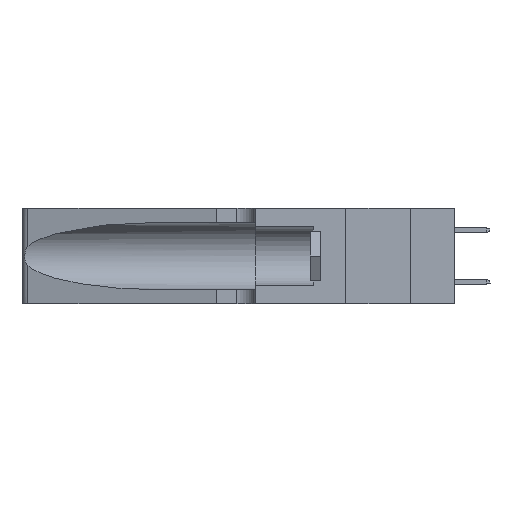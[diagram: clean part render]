
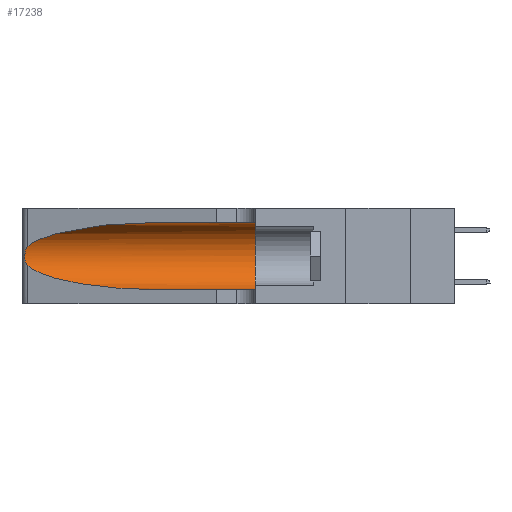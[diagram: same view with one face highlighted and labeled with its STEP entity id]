
A CAD part, left-side view. The second image highlights one B-rep face of the part: STEP entity #17238.
In plain terms, the highlighted cylindrical face has radius 3.308 mm (diameter 6.617 mm), a partial arc.
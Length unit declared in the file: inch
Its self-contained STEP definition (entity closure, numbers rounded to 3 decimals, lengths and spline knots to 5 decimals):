
#310 = CARTESIAN_POINT ( 'NONE',  ( 0.1305, 1.61858, 0.185 ) ) ;
#352 = CARTESIAN_POINT ( 'NONE',  ( 0.25487, 1.22718, 0.22369 ) ) ;
#636 = DIRECTION ( 'NONE',  ( 0., 1., 0. ) ) ;
#2686 = DIRECTION ( 'NONE',  ( 0., 0., 1. ) ) ;
#3085 = EDGE_CURVE ( 'NONE', #28419, #7694, #16352, .T. ) ;
#3163 = EDGE_LOOP ( 'NONE', ( #8327, #13606, #5145, #22770, #24645, #8118 ) ) ;
#3360 = CARTESIAN_POINT ( 'NONE',  ( 0.26075, 1.23896, 0.178 ) ) ;
#3658 = CARTESIAN_POINT ( 'NONE',  ( 0.25487, 1.22718, 0.22369 ) ) ;
#3669 = AXIS2_PLACEMENT_3D ( 'NONE', #310, #9234, #22348 ) ;
#4435 = CARTESIAN_POINT ( 'NONE',  ( 0.25487, 1.22718, 0.14631 ) ) ;
#5102 = EDGE_CURVE ( 'NONE', #12099, #28419, #13358, .T. ) ;
#5145 = ORIENTED_EDGE ( 'NONE', *, *, #10471, .T. ) ;
#7182 = CARTESIAN_POINT ( 'NONE',  ( 0.25555, 1.22994, 0.2215 ) ) ;
#7206 = CARTESIAN_POINT ( 'NONE',  ( 0.1305, 0.35, 0.185 ) ) ;
#7694 = VERTEX_POINT ( 'NONE', #22421 ) ;
#7907 = CARTESIAN_POINT ( 'NONE',  ( 0.1305, 0.72297, 0.31525 ) ) ;
#8118 = ORIENTED_EDGE ( 'NONE', *, *, #5102, .F. ) ;
#8327 = ORIENTED_EDGE ( 'NONE', *, *, #25063, .T. ) ;
#8345 = VECTOR ( 'NONE', #12967, 39.37008 ) ;
#9234 = DIRECTION ( 'NONE',  ( 0., -1., 0. ) ) ;
#9275 = EDGE_CURVE ( 'NONE', #16780, #10342, #11968, .T. ) ;
#9394 = CARTESIAN_POINT ( 'NONE',  ( 0.25487, 1.22718, 0.14631 ) ) ;
#9401 = CARTESIAN_POINT ( 'NONE',  ( 0.25487, 1.22718, 0.22369 ) ) ;
#10110 = CARTESIAN_POINT ( 'NONE',  ( 0.26075, 1.23896, 0.19203 ) ) ;
#10342 = VERTEX_POINT ( 'NONE', #28223 ) ;
#10471 = EDGE_CURVE ( 'NONE', #10342, #26490, #19656, .T. ) ;
#11968 = B_SPLINE_CURVE_WITH_KNOTS ( 'NONE', 3,
 ( #9401, #7182, #14020, #18959, #14452, #23371, #10110, #3360, #27914, #12275, #18146, #15939, #22121, #4435 ),
 .UNSPECIFIED., .F., .F.,
 ( 4, 2, 2, 2, 2, 2, 4 ),
 ( 0., 0.00027, 0.00053, 0.00107, 0.0016, 0.00187, 0.00214 ),
 .UNSPECIFIED. ) ;
#12099 = VERTEX_POINT ( 'NONE', #7907 ) ;
#12275 = CARTESIAN_POINT ( 'NONE',  ( 0.25856, 1.23593, 0.16098 ) ) ;
#12567 = CARTESIAN_POINT ( 'NONE',  ( 0.1305, 0.72297, 0.31525 ) ) ;
#12763 =( BOUNDED_CURVE ( )  B_SPLINE_CURVE ( 3, ( #12567, #28210, #28356, #3658 ),
 .UNSPECIFIED., .F., .T. ) 
 B_SPLINE_CURVE_WITH_KNOTS ( ( 4, 4 ),
 ( 1.5708, 2.84003 ),
 .UNSPECIFIED. ) 
 CURVE ( )  GEOMETRIC_REPRESENTATION_ITEM ( )  RATIONAL_B_SPLINE_CURVE ( ( 1., 0.87, 0.87, 1. ) ) 
 REPRESENTATION_ITEM ( '' )  );
#12967 = DIRECTION ( 'NONE',  ( 0., -1., 0. ) ) ;
#13121 = LINE ( 'NONE', #28623, #8345 ) ;
#13358 = LINE ( 'NONE', #15959, #15844 ) ;
#13432 = CYLINDRICAL_SURFACE ( 'NONE', #3669, 0.13025 ) ;
#13606 = ORIENTED_EDGE ( 'NONE', *, *, #9275, .T. ) ;
#14020 = CARTESIAN_POINT ( 'NONE',  ( 0.25639, 1.23184, 0.21858 ) ) ;
#14452 = CARTESIAN_POINT ( 'NONE',  ( 0.25854, 1.2359, 0.20912 ) ) ;
#15586 = CARTESIAN_POINT ( 'NONE',  ( 0.1305, 0.35, 0.31525 ) ) ;
#15844 = VECTOR ( 'NONE', #27120, 39.37008 ) ;
#15939 = CARTESIAN_POINT ( 'NONE',  ( 0.25639, 1.23186, 0.15144 ) ) ;
#15959 = CARTESIAN_POINT ( 'NONE',  ( 0.1305, 1.61858, 0.31525 ) ) ;
#16352 = CIRCLE ( 'NONE', #27566, 0.13025 ) ;
#16780 = VERTEX_POINT ( 'NONE', #352 ) ;
#17238 = ADVANCED_FACE ( 'NONE', ( #24991 ), #13432, .F. ) ;
#18107 = CARTESIAN_POINT ( 'NONE',  ( 0.2373, 1.15595, 0.08982 ) ) ;
#18146 = CARTESIAN_POINT ( 'NONE',  ( 0.25789, 1.23486, 0.15765 ) ) ;
#18251 = CARTESIAN_POINT ( 'NONE',  ( 0.18966, 0.96281, 0.05475 ) ) ;
#18872 = EDGE_CURVE ( 'NONE', #26490, #7694, #13121, .T. ) ;
#18959 = CARTESIAN_POINT ( 'NONE',  ( 0.25787, 1.23484, 0.2124 ) ) ;
#19656 =( BOUNDED_CURVE ( )  B_SPLINE_CURVE ( 3, ( #9394, #18107, #18251, #27198 ),
 .UNSPECIFIED., .F., .T. ) 
 B_SPLINE_CURVE_WITH_KNOTS ( ( 4, 4 ),
 ( 3.44316, 4.71239 ),
 .UNSPECIFIED. ) 
 CURVE ( )  GEOMETRIC_REPRESENTATION_ITEM ( )  RATIONAL_B_SPLINE_CURVE ( ( 1., 0.87, 0.87, 1. ) ) 
 REPRESENTATION_ITEM ( '' )  );
#22121 = CARTESIAN_POINT ( 'NONE',  ( 0.25555, 1.22993, 0.14849 ) ) ;
#22348 = DIRECTION ( 'NONE',  ( 0., 0., -1. ) ) ;
#22421 = CARTESIAN_POINT ( 'NONE',  ( 0.1305, 0.35, 0.05475 ) ) ;
#22770 = ORIENTED_EDGE ( 'NONE', *, *, #18872, .T. ) ;
#23371 = CARTESIAN_POINT ( 'NONE',  ( 0.26018, 1.23835, 0.19895 ) ) ;
#24645 = ORIENTED_EDGE ( 'NONE', *, *, #3085, .F. ) ;
#24991 = FACE_OUTER_BOUND ( 'NONE', #3163, .T. ) ;
#25063 = EDGE_CURVE ( 'NONE', #12099, #16780, #12763, .T. ) ;
#25876 = CARTESIAN_POINT ( 'NONE',  ( 0.1305, 0.72297, 0.05475 ) ) ;
#26490 = VERTEX_POINT ( 'NONE', #25876 ) ;
#27120 = DIRECTION ( 'NONE',  ( 0., -1., 0. ) ) ;
#27198 = CARTESIAN_POINT ( 'NONE',  ( 0.1305, 0.72297, 0.05475 ) ) ;
#27566 = AXIS2_PLACEMENT_3D ( 'NONE', #7206, #636, #2686 ) ;
#27914 = CARTESIAN_POINT ( 'NONE',  ( 0.26017, 1.23833, 0.17102 ) ) ;
#28210 = CARTESIAN_POINT ( 'NONE',  ( 0.18966, 0.96281, 0.31525 ) ) ;
#28223 = CARTESIAN_POINT ( 'NONE',  ( 0.25487, 1.22718, 0.14631 ) ) ;
#28356 = CARTESIAN_POINT ( 'NONE',  ( 0.2373, 1.15595, 0.28018 ) ) ;
#28419 = VERTEX_POINT ( 'NONE', #15586 ) ;
#28623 = CARTESIAN_POINT ( 'NONE',  ( 0.1305, 1.61858, 0.05475 ) ) ;
